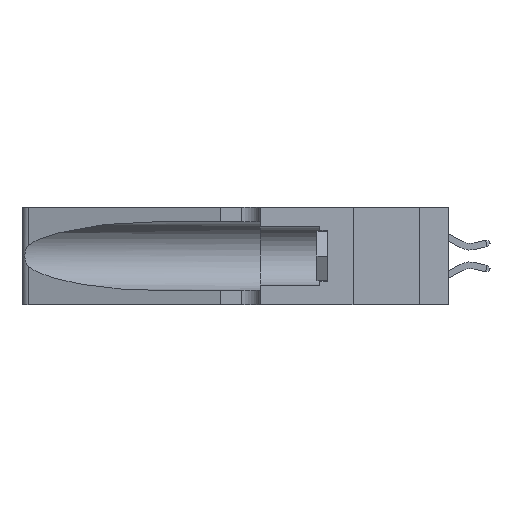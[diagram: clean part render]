
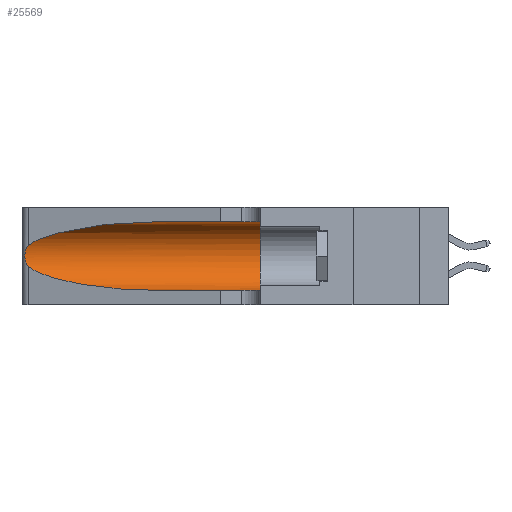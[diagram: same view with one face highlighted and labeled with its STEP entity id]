
A CAD part, left-side view. The second image highlights one B-rep face of the part: STEP entity #25569.
In plain terms, the highlighted cylindrical face has radius 3.308 mm (diameter 6.617 mm), a partial arc.
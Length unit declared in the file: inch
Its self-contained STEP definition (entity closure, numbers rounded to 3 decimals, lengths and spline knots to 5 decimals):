
#443 = VECTOR ( 'NONE', #32161, 39.37008 ) ;
#579 = CARTESIAN_POINT ( 'NONE',  ( 0.26017, 1.23833, 0.17102 ) ) ;
#722 = CARTESIAN_POINT ( 'NONE',  ( 0.25555, 1.22993, 0.14849 ) ) ;
#1206 = FACE_OUTER_BOUND ( 'NONE', #1547, .T. ) ;
#1547 = EDGE_LOOP ( 'NONE', ( #7388, #15479, #7469, #2158, #14995, #9124 ) ) ;
#2158 = ORIENTED_EDGE ( 'NONE', *, *, #6644, .T. ) ;
#2721 = CARTESIAN_POINT ( 'NONE',  ( 0.26075, 1.23896, 0.178 ) ) ;
#2780 = VERTEX_POINT ( 'NONE', #3094 ) ;
#2913 = CARTESIAN_POINT ( 'NONE',  ( 0.1305, 0.35, 0.185 ) ) ;
#3094 = CARTESIAN_POINT ( 'NONE',  ( 0.25487, 1.22718, 0.22369 ) ) ;
#3515 = EDGE_CURVE ( 'NONE', #31812, #17541, #27118, .T. ) ;
#4931 = CARTESIAN_POINT ( 'NONE',  ( 0.1305, 1.61858, 0.31525 ) ) ;
#6644 = EDGE_CURVE ( 'NONE', #17541, #20072, #26933, .T. ) ;
#7388 = ORIENTED_EDGE ( 'NONE', *, *, #13932, .T. ) ;
#7469 = ORIENTED_EDGE ( 'NONE', *, *, #3515, .T. ) ;
#7582 = CARTESIAN_POINT ( 'NONE',  ( 0.25487, 1.22718, 0.14631 ) ) ;
#7620 = CARTESIAN_POINT ( 'NONE',  ( 0.25639, 1.23184, 0.21858 ) ) ;
#7717 = DIRECTION ( 'NONE',  ( 0., 1., 0. ) ) ;
#8086 = CARTESIAN_POINT ( 'NONE',  ( 0.1305, 0.72297, 0.05475 ) ) ;
#8698 = LINE ( 'NONE', #4931, #443 ) ;
#9124 = ORIENTED_EDGE ( 'NONE', *, *, #30489, .F. ) ;
#9206 = CARTESIAN_POINT ( 'NONE',  ( 0.25487, 1.22718, 0.22369 ) ) ;
#9717 = DIRECTION ( 'NONE',  ( 0., -1., 0. ) ) ;
#10485 = CARTESIAN_POINT ( 'NONE',  ( 0.25487, 1.22718, 0.14631 ) ) ;
#11973 = CARTESIAN_POINT ( 'NONE',  ( 0.2373, 1.15595, 0.28018 ) ) ;
#12014 = EDGE_CURVE ( 'NONE', #2780, #31812, #26893, .T. ) ;
#12057 = EDGE_CURVE ( 'NONE', #15427, #20072, #23852, .T. ) ;
#12624 = CARTESIAN_POINT ( 'NONE',  ( 0.26075, 1.23896, 0.19203 ) ) ;
#12633 = AXIS2_PLACEMENT_3D ( 'NONE', #19951, #9717, #17341 ) ;
#12846 = CARTESIAN_POINT ( 'NONE',  ( 0.25856, 1.23593, 0.16098 ) ) ;
#13022 = CARTESIAN_POINT ( 'NONE',  ( 0.2373, 1.15595, 0.08982 ) ) ;
#13352 = CARTESIAN_POINT ( 'NONE',  ( 0.18966, 0.96281, 0.05475 ) ) ;
#13621 = CARTESIAN_POINT ( 'NONE',  ( 0.25487, 1.22718, 0.14631 ) ) ;
#13932 = EDGE_CURVE ( 'NONE', #31626, #2780, #17669, .T. ) ;
#14344 = CARTESIAN_POINT ( 'NONE',  ( 0.1305, 0.35, 0.31525 ) ) ;
#14995 = ORIENTED_EDGE ( 'NONE', *, *, #12057, .F. ) ;
#15427 = VERTEX_POINT ( 'NONE', #14344 ) ;
#15479 = ORIENTED_EDGE ( 'NONE', *, *, #12014, .T. ) ;
#17341 = DIRECTION ( 'NONE',  ( 0., 0., -1. ) ) ;
#17452 = CARTESIAN_POINT ( 'NONE',  ( 0.25787, 1.23484, 0.2124 ) ) ;
#17541 = VERTEX_POINT ( 'NONE', #28844 ) ;
#17669 =( BOUNDED_CURVE ( )  B_SPLINE_CURVE ( 3, ( #21281, #26953, #11973, #29439 ),
 .UNSPECIFIED., .F., .T. ) 
 B_SPLINE_CURVE_WITH_KNOTS ( ( 4, 4 ),
 ( 1.5708, 2.84003 ),
 .UNSPECIFIED. ) 
 CURVE ( )  GEOMETRIC_REPRESENTATION_ITEM ( )  RATIONAL_B_SPLINE_CURVE ( ( 1., 0.87, 0.87, 1. ) ) 
 REPRESENTATION_ITEM ( '' )  );
#19951 = CARTESIAN_POINT ( 'NONE',  ( 0.1305, 1.61858, 0.185 ) ) ;
#20072 = VERTEX_POINT ( 'NONE', #22098 ) ;
#21281 = CARTESIAN_POINT ( 'NONE',  ( 0.1305, 0.72297, 0.31525 ) ) ;
#21589 = DIRECTION ( 'NONE',  ( 0., -1., 0. ) ) ;
#22098 = CARTESIAN_POINT ( 'NONE',  ( 0.1305, 0.35, 0.05475 ) ) ;
#22623 = VECTOR ( 'NONE', #21589, 39.37008 ) ;
#22871 = CARTESIAN_POINT ( 'NONE',  ( 0.25789, 1.23486, 0.15765 ) ) ;
#23852 = CIRCLE ( 'NONE', #24111, 0.13025 ) ;
#24111 = AXIS2_PLACEMENT_3D ( 'NONE', #2913, #7717, #27800 ) ;
#24568 = CARTESIAN_POINT ( 'NONE',  ( 0.1305, 0.72297, 0.31525 ) ) ;
#25035 = CARTESIAN_POINT ( 'NONE',  ( 0.25854, 1.2359, 0.20912 ) ) ;
#25477 = CARTESIAN_POINT ( 'NONE',  ( 0.1305, 1.61858, 0.05475 ) ) ;
#25569 = ADVANCED_FACE ( 'NONE', ( #1206 ), #25777, .F. ) ;
#25777 = CYLINDRICAL_SURFACE ( 'NONE', #12633, 0.13025 ) ;
#26893 = B_SPLINE_CURVE_WITH_KNOTS ( 'NONE', 3,
 ( #9206, #29163, #7620, #17452, #25035, #27595, #12624, #2721, #579, #12846, #22871, #31020, #722, #13621 ),
 .UNSPECIFIED., .F., .F.,
 ( 4, 2, 2, 2, 2, 2, 4 ),
 ( 0., 0.00027, 0.00053, 0.00107, 0.0016, 0.00187, 0.00214 ),
 .UNSPECIFIED. ) ;
#26933 = LINE ( 'NONE', #25477, #22623 ) ;
#26953 = CARTESIAN_POINT ( 'NONE',  ( 0.18966, 0.96281, 0.31525 ) ) ;
#27118 =( BOUNDED_CURVE ( )  B_SPLINE_CURVE ( 3, ( #10485, #13022, #13352, #8086 ),
 .UNSPECIFIED., .F., .T. ) 
 B_SPLINE_CURVE_WITH_KNOTS ( ( 4, 4 ),
 ( 3.44316, 4.71239 ),
 .UNSPECIFIED. ) 
 CURVE ( )  GEOMETRIC_REPRESENTATION_ITEM ( )  RATIONAL_B_SPLINE_CURVE ( ( 1., 0.87, 0.87, 1. ) ) 
 REPRESENTATION_ITEM ( '' )  );
#27595 = CARTESIAN_POINT ( 'NONE',  ( 0.26018, 1.23835, 0.19895 ) ) ;
#27800 = DIRECTION ( 'NONE',  ( 0., 0., 1. ) ) ;
#28844 = CARTESIAN_POINT ( 'NONE',  ( 0.1305, 0.72297, 0.05475 ) ) ;
#29163 = CARTESIAN_POINT ( 'NONE',  ( 0.25555, 1.22994, 0.2215 ) ) ;
#29439 = CARTESIAN_POINT ( 'NONE',  ( 0.25487, 1.22718, 0.22369 ) ) ;
#30489 = EDGE_CURVE ( 'NONE', #31626, #15427, #8698, .T. ) ;
#31020 = CARTESIAN_POINT ( 'NONE',  ( 0.25639, 1.23186, 0.15144 ) ) ;
#31626 = VERTEX_POINT ( 'NONE', #24568 ) ;
#31812 = VERTEX_POINT ( 'NONE', #7582 ) ;
#32161 = DIRECTION ( 'NONE',  ( 0., -1., 0. ) ) ;
